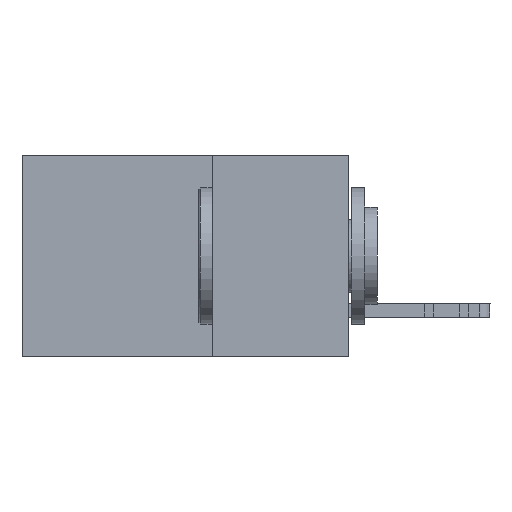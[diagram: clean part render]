
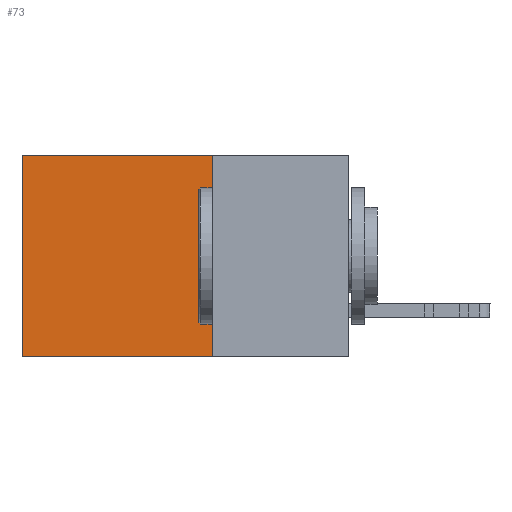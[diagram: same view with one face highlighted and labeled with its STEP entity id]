
A CAD part, left-side view. The second image highlights one B-rep face of the part: STEP entity #73.
In plain terms, the highlighted planar face has unit normal (-1, 0, 0).
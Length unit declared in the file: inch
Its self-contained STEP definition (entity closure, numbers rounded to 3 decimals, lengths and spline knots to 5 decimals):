
#73 = ADVANCED_FACE ( 'NONE', ( #18192 ), #17933, .F. ) ;
#445 = DIRECTION ( 'NONE',  ( 0., 0., -1. ) ) ;
#3950 = ORIENTED_EDGE ( 'NONE', *, *, #11474, .T. ) ;
#4402 = ORIENTED_EDGE ( 'NONE', *, *, #29170, .T. ) ;
#6118 = VECTOR ( 'NONE', #21174, 39.37008 ) ;
#6978 = CARTESIAN_POINT ( 'NONE',  ( 0.298, 0.25, 0. ) ) ;
#8389 = VERTEX_POINT ( 'NONE', #24351 ) ;
#9039 = CARTESIAN_POINT ( 'NONE',  ( 0.298, 0.6, -0.37 ) ) ;
#9267 = DIRECTION ( 'NONE',  ( 0., 1., 0. ) ) ;
#10611 = LINE ( 'NONE', #19042, #6118 ) ;
#10792 = VERTEX_POINT ( 'NONE', #13182 ) ;
#10870 = DIRECTION ( 'NONE',  ( 1., 0., 0. ) ) ;
#11188 = ORIENTED_EDGE ( 'NONE', *, *, #20700, .F. ) ;
#11266 = CARTESIAN_POINT ( 'NONE',  ( 0.298, 0.25, 0. ) ) ;
#11474 = EDGE_CURVE ( 'NONE', #23218, #19254, #29283, .T. ) ;
#13182 = CARTESIAN_POINT ( 'NONE',  ( 0.298, 0.25, 0. ) ) ;
#14983 = AXIS2_PLACEMENT_3D ( 'NONE', #11266, #10870, #27337 ) ;
#15298 = LINE ( 'NONE', #16732, #25576 ) ;
#16732 = CARTESIAN_POINT ( 'NONE',  ( 0.298, 0.25, 0. ) ) ;
#17933 = PLANE ( 'NONE',  #14983 ) ;
#18192 = FACE_OUTER_BOUND ( 'NONE', #26120, .T. ) ;
#19042 = CARTESIAN_POINT ( 'NONE',  ( 0.298, 0.25, -0.37 ) ) ;
#19254 = VERTEX_POINT ( 'NONE', #9039 ) ;
#20700 = EDGE_CURVE ( 'NONE', #8389, #19254, #10611, .T. ) ;
#21174 = DIRECTION ( 'NONE',  ( 0., 1., 0. ) ) ;
#22580 = CARTESIAN_POINT ( 'NONE',  ( 0.298, 0.6, 0. ) ) ;
#23218 = VERTEX_POINT ( 'NONE', #22580 ) ;
#23329 = LINE ( 'NONE', #6978, #27064 ) ;
#23875 = CARTESIAN_POINT ( 'NONE',  ( 0.298, 0.6, 0. ) ) ;
#24191 = DIRECTION ( 'NONE',  ( 0., 0., -1. ) ) ;
#24351 = CARTESIAN_POINT ( 'NONE',  ( 0.298, 0.25, -0.37 ) ) ;
#24820 = VECTOR ( 'NONE', #24191, 39.37008 ) ;
#25576 = VECTOR ( 'NONE', #445, 39.37008 ) ;
#26120 = EDGE_LOOP ( 'NONE', ( #3950, #11188, #29558, #4402 ) ) ;
#27064 = VECTOR ( 'NONE', #9267, 39.37008 ) ;
#27337 = DIRECTION ( 'NONE',  ( 0., 0., -1. ) ) ;
#29170 = EDGE_CURVE ( 'NONE', #10792, #23218, #23329, .T. ) ;
#29283 = LINE ( 'NONE', #23875, #24820 ) ;
#29558 = ORIENTED_EDGE ( 'NONE', *, *, #29905, .F. ) ;
#29905 = EDGE_CURVE ( 'NONE', #10792, #8389, #15298, .T. ) ;
